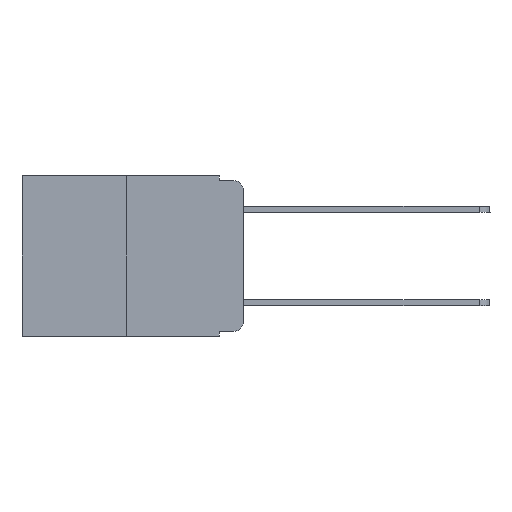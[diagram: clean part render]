
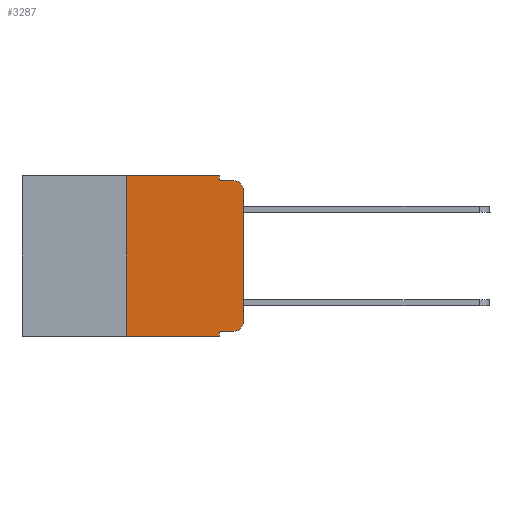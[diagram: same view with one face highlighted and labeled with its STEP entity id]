
A CAD part, left-side view. The second image highlights one B-rep face of the part: STEP entity #3287.
In plain terms, the highlighted planar face has unit normal (-1, 0, 0).
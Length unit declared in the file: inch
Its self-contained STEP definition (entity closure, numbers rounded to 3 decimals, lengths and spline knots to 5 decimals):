
#51 = EDGE_LOOP ( 'NONE', ( #8088, #3388, #8517, #3941, #10615, #4700, #12050, #9970, #9399, #11702 ) ) ;
#87 = CARTESIAN_POINT ( 'NONE',  ( 0., 0.473, 0. ) ) ;
#752 = EDGE_CURVE ( 'NONE', #11088, #9665, #9373, .T. ) ;
#768 = LINE ( 'NONE', #8844, #9807 ) ;
#839 = AXIS2_PLACEMENT_3D ( 'NONE', #87, #7693, #11412 ) ;
#898 = VERTEX_POINT ( 'NONE', #3148 ) ;
#913 = CARTESIAN_POINT ( 'NONE',  ( 0., 0.051, 0. ) ) ;
#1022 = VECTOR ( 'NONE', #8917, 39.37008 ) ;
#1438 = CARTESIAN_POINT ( 'NONE',  ( 0., 0., 0. ) ) ;
#1477 = VECTOR ( 'NONE', #5533, 39.37008 ) ;
#1678 = CARTESIAN_POINT ( 'NONE',  ( 0., 0.051, -0.333 ) ) ;
#1876 = LINE ( 'NONE', #913, #4358 ) ;
#2089 = CARTESIAN_POINT ( 'NONE',  ( 0., 0.25, 0. ) ) ;
#2173 = CARTESIAN_POINT ( 'NONE',  ( 0., 0.051, -0.01 ) ) ;
#2407 = CARTESIAN_POINT ( 'NONE',  ( 0., 0.02, -0.01 ) ) ;
#3120 = EDGE_CURVE ( 'NONE', #11273, #10313, #11063, .T. ) ;
#3148 = CARTESIAN_POINT ( 'NONE',  ( 0., 0., -0.313 ) ) ;
#3287 = ADVANCED_FACE ( 'NONE', ( #6542 ), #6725, .F. ) ;
#3295 = CIRCLE ( 'NONE', #10495, 0.02 ) ;
#3388 = ORIENTED_EDGE ( 'NONE', *, *, #11059, .T. ) ;
#3432 = CARTESIAN_POINT ( 'NONE',  ( 0., 0.051, 0. ) ) ;
#3650 = CARTESIAN_POINT ( 'NONE',  ( 0., 0.02, -0.03 ) ) ;
#3675 = VERTEX_POINT ( 'NONE', #6342 ) ;
#3740 = VERTEX_POINT ( 'NONE', #5782 ) ;
#3893 = DIRECTION ( 'NONE',  ( 0., 0., -1. ) ) ;
#3941 = ORIENTED_EDGE ( 'NONE', *, *, #5861, .F. ) ;
#4270 = EDGE_CURVE ( 'NONE', #4682, #7026, #9487, .T. ) ;
#4358 = VECTOR ( 'NONE', #5525, 39.37008 ) ;
#4420 = DIRECTION ( 'NONE',  ( 0., 0., 1. ) ) ;
#4462 = EDGE_CURVE ( 'NONE', #898, #3675, #10828, .T. ) ;
#4682 = VERTEX_POINT ( 'NONE', #2089 ) ;
#4700 = ORIENTED_EDGE ( 'NONE', *, *, #8375, .F. ) ;
#5032 = DIRECTION ( 'NONE',  ( 0., -1., 0. ) ) ;
#5525 = DIRECTION ( 'NONE',  ( 0., 0., -1. ) ) ;
#5533 = DIRECTION ( 'NONE',  ( 0., -1., 0. ) ) ;
#5680 = CARTESIAN_POINT ( 'NONE',  ( 0., 0.051, 0. ) ) ;
#5782 = CARTESIAN_POINT ( 'NONE',  ( 0., 0.051, -0.343 ) ) ;
#5788 = VECTOR ( 'NONE', #7574, 39.37008 ) ;
#5861 = EDGE_CURVE ( 'NONE', #7026, #11088, #1876, .T. ) ;
#6025 = AXIS2_PLACEMENT_3D ( 'NONE', #3650, #6512, #3893 ) ;
#6342 = CARTESIAN_POINT ( 'NONE',  ( 0., 0., -0.03 ) ) ;
#6512 = DIRECTION ( 'NONE',  ( -1., 0., 0. ) ) ;
#6542 = FACE_OUTER_BOUND ( 'NONE', #51, .T. ) ;
#6623 = CARTESIAN_POINT ( 'NONE',  ( 0., 0.02, -0.313 ) ) ;
#6724 = LINE ( 'NONE', #5680, #5788 ) ;
#6725 = PLANE ( 'NONE',  #839 ) ;
#7026 = VERTEX_POINT ( 'NONE', #3432 ) ;
#7378 = EDGE_CURVE ( 'NONE', #11273, #3740, #6724, .T. ) ;
#7394 = CARTESIAN_POINT ( 'NONE',  ( 0., 0.02, -0.333 ) ) ;
#7574 = DIRECTION ( 'NONE',  ( 0., 0., -1. ) ) ;
#7693 = DIRECTION ( 'NONE',  ( 1., 0., 0. ) ) ;
#7710 = DIRECTION ( 'NONE',  ( 0., 0., -1. ) ) ;
#8059 = DIRECTION ( 'NONE',  ( 0., -1., 0. ) ) ;
#8088 = ORIENTED_EDGE ( 'NONE', *, *, #4462, .T. ) ;
#8375 = EDGE_CURVE ( 'NONE', #11835, #4682, #768, .T. ) ;
#8458 = CARTESIAN_POINT ( 'NONE',  ( 0., 0.051, -0.01 ) ) ;
#8517 = ORIENTED_EDGE ( 'NONE', *, *, #752, .F. ) ;
#8844 = CARTESIAN_POINT ( 'NONE',  ( 0., 0.25, 0. ) ) ;
#8891 = DIRECTION ( 'NONE',  ( 0., -1., 0. ) ) ;
#8917 = DIRECTION ( 'NONE',  ( 0., 0., 1. ) ) ;
#9373 = LINE ( 'NONE', #8458, #1477 ) ;
#9399 = ORIENTED_EDGE ( 'NONE', *, *, #3120, .T. ) ;
#9487 = LINE ( 'NONE', #9547, #9745 ) ;
#9547 = CARTESIAN_POINT ( 'NONE',  ( 0., 0.473, 0. ) ) ;
#9665 = VERTEX_POINT ( 'NONE', #2407 ) ;
#9745 = VECTOR ( 'NONE', #5032, 39.37008 ) ;
#9807 = VECTOR ( 'NONE', #4420, 39.37008 ) ;
#9956 = EDGE_CURVE ( 'NONE', #10313, #898, #3295, .T. ) ;
#9970 = ORIENTED_EDGE ( 'NONE', *, *, #7378, .F. ) ;
#10104 = EDGE_CURVE ( 'NONE', #11835, #3740, #11491, .T. ) ;
#10313 = VERTEX_POINT ( 'NONE', #7394 ) ;
#10495 = AXIS2_PLACEMENT_3D ( 'NONE', #6623, #11195, #7710 ) ;
#10509 = CARTESIAN_POINT ( 'NONE',  ( 0., 0.473, -0.343 ) ) ;
#10615 = ORIENTED_EDGE ( 'NONE', *, *, #4270, .F. ) ;
#10828 = LINE ( 'NONE', #1438, #1022 ) ;
#11059 = EDGE_CURVE ( 'NONE', #3675, #9665, #11301, .T. ) ;
#11063 = LINE ( 'NONE', #1678, #11352 ) ;
#11088 = VERTEX_POINT ( 'NONE', #2173 ) ;
#11195 = DIRECTION ( 'NONE',  ( -1., 0., 0. ) ) ;
#11273 = VERTEX_POINT ( 'NONE', #11939 ) ;
#11301 = CIRCLE ( 'NONE', #6025, 0.02 ) ;
#11343 = CARTESIAN_POINT ( 'NONE',  ( 0., 0.25, -0.343 ) ) ;
#11352 = VECTOR ( 'NONE', #8059, 39.37008 ) ;
#11412 = DIRECTION ( 'NONE',  ( 0., 0., -1. ) ) ;
#11491 = LINE ( 'NONE', #10509, #11880 ) ;
#11702 = ORIENTED_EDGE ( 'NONE', *, *, #9956, .T. ) ;
#11835 = VERTEX_POINT ( 'NONE', #11343 ) ;
#11880 = VECTOR ( 'NONE', #8891, 39.37008 ) ;
#11939 = CARTESIAN_POINT ( 'NONE',  ( 0., 0.051, -0.333 ) ) ;
#12050 = ORIENTED_EDGE ( 'NONE', *, *, #10104, .T. ) ;
